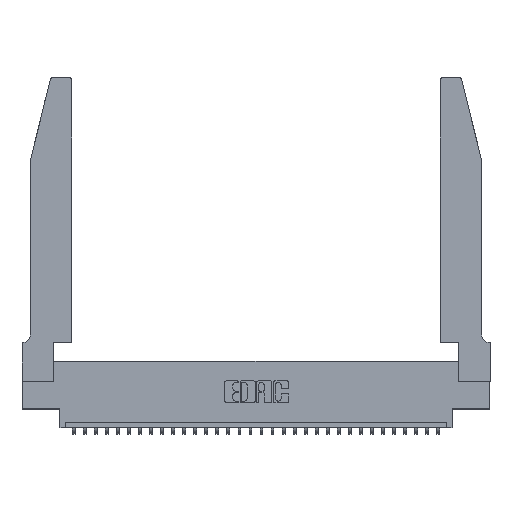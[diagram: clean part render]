
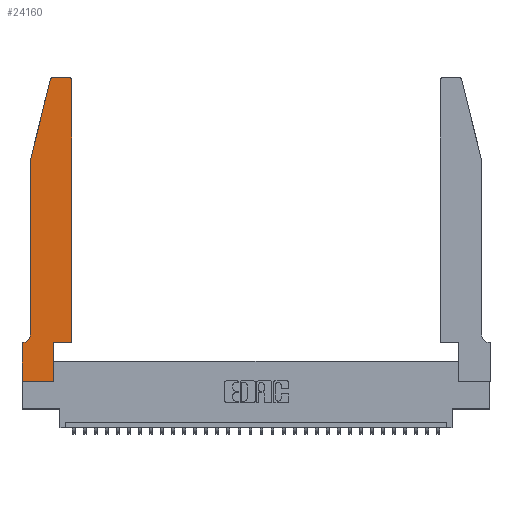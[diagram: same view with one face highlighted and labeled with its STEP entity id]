
A CAD part, top view. The second image highlights one B-rep face of the part: STEP entity #24160.
In plain terms, the highlighted planar face has unit normal (0, 0, 1).
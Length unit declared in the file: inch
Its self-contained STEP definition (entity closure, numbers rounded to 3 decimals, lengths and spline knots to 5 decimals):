
#2 = PLANE ( 'NONE',  #14602 ) ;
#806 = CARTESIAN_POINT ( 'NONE',  ( 0.25487, 2.72718, 0.37 ) ) ;
#968 = ORIENTED_EDGE ( 'NONE', *, *, #2258, .T. ) ;
#1078 = EDGE_CURVE ( 'NONE', #9675, #10535, #18708, .T. ) ;
#1277 = EDGE_CURVE ( 'NONE', #28247, #7486, #4467, .T. ) ;
#1310 = EDGE_CURVE ( 'NONE', #21303, #29317, #25536, .T. ) ;
#1417 = LINE ( 'NONE', #24546, #26619 ) ;
#1542 = CARTESIAN_POINT ( 'NONE',  ( 0.4205, 2.75, 0.37 ) ) ;
#1765 = CARTESIAN_POINT ( 'NONE',  ( 0., 0., 0.37 ) ) ;
#2258 = EDGE_CURVE ( 'NONE', #10535, #29739, #1417, .T. ) ;
#3293 = LINE ( 'NONE', #14825, #29311 ) ;
#4467 = LINE ( 'NONE', #10070, #9465 ) ;
#4784 = CARTESIAN_POINT ( 'NONE',  ( 0.4505, 0.35, 0.37 ) ) ;
#5011 = DIRECTION ( 'NONE',  ( 0., 1., 0. ) ) ;
#5103 = ORIENTED_EDGE ( 'NONE', *, *, #26405, .T. ) ;
#5276 = ORIENTED_EDGE ( 'NONE', *, *, #23075, .T. ) ;
#5414 = EDGE_CURVE ( 'NONE', #23422, #9430, #13415, .T. ) ;
#5821 = VERTEX_POINT ( 'NONE', #17763 ) ;
#5911 = ORIENTED_EDGE ( 'NONE', *, *, #1277, .T. ) ;
#6324 = EDGE_CURVE ( 'NONE', #9430, #28749, #9417, .T. ) ;
#6699 = ORIENTED_EDGE ( 'NONE', *, *, #13218, .T. ) ;
#7231 = CIRCLE ( 'NONE', #24236, 0.03 ) ;
#7367 = EDGE_LOOP ( 'NONE', ( #5911, #9784, #5103, #21270, #31124, #17273, #5276, #18011, #968, #6699, #18860, #20928 ) ) ;
#7486 = VERTEX_POINT ( 'NONE', #20174 ) ;
#8260 = VECTOR ( 'NONE', #30959, 39.37008 ) ;
#8453 = CARTESIAN_POINT ( 'NONE',  ( 0.0055, 0.42, 0.37 ) ) ;
#8522 = CARTESIAN_POINT ( 'NONE',  ( 0., 0., 0.37 ) ) ;
#8717 = CARTESIAN_POINT ( 'NONE',  ( 0.0755, 0.35, 0.37 ) ) ;
#8926 = CARTESIAN_POINT ( 'NONE',  ( 0.4505, 2.72, 0.37 ) ) ;
#9417 = LINE ( 'NONE', #8717, #15155 ) ;
#9430 = VERTEX_POINT ( 'NONE', #18817 ) ;
#9465 = VECTOR ( 'NONE', #27168, 39.37008 ) ;
#9675 = VERTEX_POINT ( 'NONE', #8522 ) ;
#9784 = ORIENTED_EDGE ( 'NONE', *, *, #25427, .T. ) ;
#9802 = DIRECTION ( 'NONE',  ( 0., 0., 1. ) ) ;
#10070 = CARTESIAN_POINT ( 'NONE',  ( 0.2605, 2.75, 0.37 ) ) ;
#10535 = VERTEX_POINT ( 'NONE', #30819 ) ;
#11575 = AXIS2_PLACEMENT_3D ( 'NONE', #12476, #9802, #17206 ) ;
#12233 = CARTESIAN_POINT ( 'NONE',  ( 0.4205, 2.72, 0.37 ) ) ;
#12437 = CIRCLE ( 'NONE', #11575, 0.03 ) ;
#12476 = CARTESIAN_POINT ( 'NONE',  ( 0.284, 2.72, 0.37 ) ) ;
#12884 = EDGE_CURVE ( 'NONE', #29317, #28247, #7231, .T. ) ;
#13218 = EDGE_CURVE ( 'NONE', #29739, #21303, #16476, .T. ) ;
#13415 = CIRCLE ( 'NONE', #27566, 0.07 ) ;
#13627 = DIRECTION ( 'NONE',  ( -0.239, -0.971, 0. ) ) ;
#14602 = AXIS2_PLACEMENT_3D ( 'NONE', #29356, #22184, #19525 ) ;
#14825 = CARTESIAN_POINT ( 'NONE',  ( 0., 0., 0.37 ) ) ;
#15155 = VECTOR ( 'NONE', #16019, 39.37008 ) ;
#15647 = DIRECTION ( 'NONE',  ( 0., 0., 1. ) ) ;
#15769 = EDGE_CURVE ( 'NONE', #5821, #23422, #18256, .T. ) ;
#16019 = DIRECTION ( 'NONE',  ( -1., 0., 0. ) ) ;
#16476 = LINE ( 'NONE', #27091, #31009 ) ;
#17206 = DIRECTION ( 'NONE',  ( 1., 0., 0. ) ) ;
#17273 = ORIENTED_EDGE ( 'NONE', *, *, #6324, .T. ) ;
#17763 = CARTESIAN_POINT ( 'NONE',  ( 0.0755, 2., 0.37 ) ) ;
#17794 = DIRECTION ( 'NONE',  ( 1., 0., 0. ) ) ;
#18011 = ORIENTED_EDGE ( 'NONE', *, *, #1078, .T. ) ;
#18256 = LINE ( 'NONE', #23257, #8260 ) ;
#18708 = LINE ( 'NONE', #1765, #29755 ) ;
#18817 = CARTESIAN_POINT ( 'NONE',  ( 0.0055, 0.35, 0.37 ) ) ;
#18860 = ORIENTED_EDGE ( 'NONE', *, *, #1310, .T. ) ;
#19131 = VERTEX_POINT ( 'NONE', #806 ) ;
#19361 = FACE_OUTER_BOUND ( 'NONE', #7367, .T. ) ;
#19525 = DIRECTION ( 'NONE',  ( 1., 0., 0. ) ) ;
#20174 = CARTESIAN_POINT ( 'NONE',  ( 0.284, 2.75, 0.37 ) ) ;
#20647 = DIRECTION ( 'NONE',  ( -1., 0., 0. ) ) ;
#20928 = ORIENTED_EDGE ( 'NONE', *, *, #12884, .T. ) ;
#21270 = ORIENTED_EDGE ( 'NONE', *, *, #15769, .T. ) ;
#21303 = VERTEX_POINT ( 'NONE', #29176 ) ;
#21322 = DIRECTION ( 'NONE',  ( 1., 0., 0. ) ) ;
#21590 = VECTOR ( 'NONE', #13627, 39.37008 ) ;
#21732 = VECTOR ( 'NONE', #5011, 39.37008 ) ;
#21797 = DIRECTION ( 'NONE',  ( 0., 1., 0. ) ) ;
#22184 = DIRECTION ( 'NONE',  ( 0., 0., 1. ) ) ;
#23075 = EDGE_CURVE ( 'NONE', #28749, #9675, #3293, .T. ) ;
#23257 = CARTESIAN_POINT ( 'NONE',  ( 0.0755, 2., 0.37 ) ) ;
#23327 = CARTESIAN_POINT ( 'NONE',  ( 0., 0.35, 0.37 ) ) ;
#23422 = VERTEX_POINT ( 'NONE', #29431 ) ;
#23536 = LINE ( 'NONE', #25693, #21590 ) ;
#24160 = ADVANCED_FACE ( 'NONE', ( #19361 ), #2, .T. ) ;
#24236 = AXIS2_PLACEMENT_3D ( 'NONE', #12233, #15647, #17794 ) ;
#24546 = CARTESIAN_POINT ( 'NONE',  ( 0.2865, 0.35, 0.37 ) ) ;
#25427 = EDGE_CURVE ( 'NONE', #7486, #19131, #12437, .T. ) ;
#25536 = LINE ( 'NONE', #4784, #21732 ) ;
#25693 = CARTESIAN_POINT ( 'NONE',  ( 0.0755, 2., 0.37 ) ) ;
#26405 = EDGE_CURVE ( 'NONE', #19131, #5821, #23536, .T. ) ;
#26619 = VECTOR ( 'NONE', #21797, 39.37008 ) ;
#26790 = DIRECTION ( 'NONE',  ( 0., -1., 0. ) ) ;
#26951 = CARTESIAN_POINT ( 'NONE',  ( 0.2865, 0.35, 0.37 ) ) ;
#27091 = CARTESIAN_POINT ( 'NONE',  ( 0.4505, 0.35, 0.37 ) ) ;
#27168 = DIRECTION ( 'NONE',  ( -1., 0., 0. ) ) ;
#27566 = AXIS2_PLACEMENT_3D ( 'NONE', #8453, #30172, #20647 ) ;
#28247 = VERTEX_POINT ( 'NONE', #1542 ) ;
#28749 = VERTEX_POINT ( 'NONE', #23327 ) ;
#29176 = CARTESIAN_POINT ( 'NONE',  ( 0.4505, 0.35, 0.37 ) ) ;
#29311 = VECTOR ( 'NONE', #26790, 39.37008 ) ;
#29317 = VERTEX_POINT ( 'NONE', #8926 ) ;
#29356 = CARTESIAN_POINT ( 'NONE',  ( 0., 0.35, 0.37 ) ) ;
#29431 = CARTESIAN_POINT ( 'NONE',  ( 0.0755, 0.42, 0.37 ) ) ;
#29562 = DIRECTION ( 'NONE',  ( 1., 0., 0. ) ) ;
#29739 = VERTEX_POINT ( 'NONE', #26951 ) ;
#29755 = VECTOR ( 'NONE', #21322, 39.37008 ) ;
#30172 = DIRECTION ( 'NONE',  ( 0., 0., -1. ) ) ;
#30819 = CARTESIAN_POINT ( 'NONE',  ( 0.2865, 0., 0.37 ) ) ;
#30959 = DIRECTION ( 'NONE',  ( 0., -1., 0. ) ) ;
#31009 = VECTOR ( 'NONE', #29562, 39.37008 ) ;
#31124 = ORIENTED_EDGE ( 'NONE', *, *, #5414, .T. ) ;
